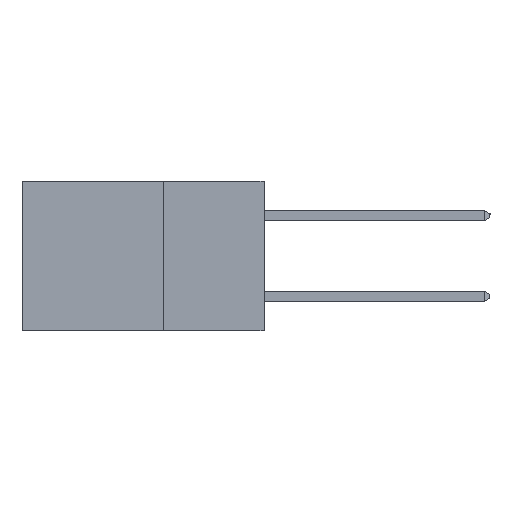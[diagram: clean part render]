
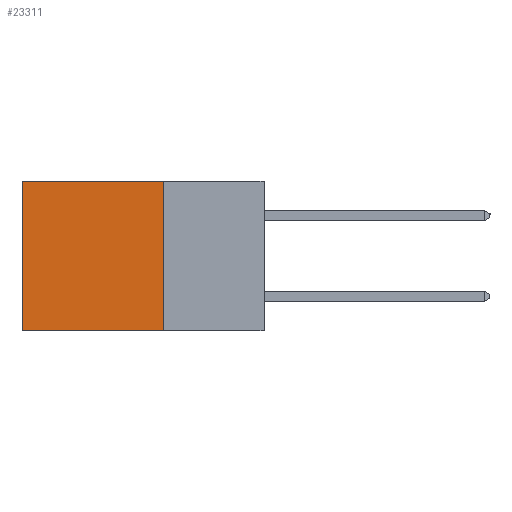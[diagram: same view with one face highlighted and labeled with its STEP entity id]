
A CAD part, left-side view. The second image highlights one B-rep face of the part: STEP entity #23311.
In plain terms, the highlighted planar face has unit normal (-1, 0, 0).
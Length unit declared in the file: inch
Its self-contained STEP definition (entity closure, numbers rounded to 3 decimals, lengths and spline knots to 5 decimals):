
#424 = CARTESIAN_POINT ( 'NONE',  ( 0.2615, 0.25, -0.37 ) ) ;
#1239 = LINE ( 'NONE', #14139, #22693 ) ;
#2942 = AXIS2_PLACEMENT_3D ( 'NONE', #22313, #9409, #12639 ) ;
#3523 = VERTEX_POINT ( 'NONE', #3964 ) ;
#3964 = CARTESIAN_POINT ( 'NONE',  ( 0.2615, 0.6, -0.37 ) ) ;
#5499 = ORIENTED_EDGE ( 'NONE', *, *, #8845, .T. ) ;
#5873 = EDGE_CURVE ( 'NONE', #17160, #3523, #1239, .T. ) ;
#6021 = LINE ( 'NONE', #424, #23474 ) ;
#7053 = DIRECTION ( 'NONE',  ( 0., 1., 0. ) ) ;
#8845 = EDGE_CURVE ( 'NONE', #20642, #14794, #18087, .T. ) ;
#8939 = PLANE ( 'NONE',  #2942 ) ;
#9409 = DIRECTION ( 'NONE',  ( 1., 0., 0. ) ) ;
#9886 = DIRECTION ( 'NONE',  ( 0., 0., -1. ) ) ;
#9913 = CARTESIAN_POINT ( 'NONE',  ( 0.2615, 0.25, -0.37 ) ) ;
#11839 = DIRECTION ( 'NONE',  ( 0., 0., -1. ) ) ;
#12007 = LINE ( 'NONE', #15729, #19194 ) ;
#12263 = EDGE_CURVE ( 'NONE', #20642, #17160, #6021, .T. ) ;
#12330 = ORIENTED_EDGE ( 'NONE', *, *, #13240, .T. ) ;
#12508 = CARTESIAN_POINT ( 'NONE',  ( 0.2615, 0.25, 0. ) ) ;
#12639 = DIRECTION ( 'NONE',  ( 0., 0., -1. ) ) ;
#13212 = VECTOR ( 'NONE', #7053, 39.37008 ) ;
#13240 = EDGE_CURVE ( 'NONE', #14794, #3523, #12007, .T. ) ;
#13629 = ORIENTED_EDGE ( 'NONE', *, *, #12263, .F. ) ;
#14024 = DIRECTION ( 'NONE',  ( 0., 1., 0. ) ) ;
#14139 = CARTESIAN_POINT ( 'NONE',  ( 0.2615, 0.25, -0.37 ) ) ;
#14794 = VERTEX_POINT ( 'NONE', #19844 ) ;
#15729 = CARTESIAN_POINT ( 'NONE',  ( 0.2615, 0.6, -0.37 ) ) ;
#17160 = VERTEX_POINT ( 'NONE', #9913 ) ;
#17414 = EDGE_LOOP ( 'NONE', ( #12330, #23998, #13629, #5499 ) ) ;
#18087 = LINE ( 'NONE', #12508, #13212 ) ;
#19194 = VECTOR ( 'NONE', #9886, 39.37008 ) ;
#19844 = CARTESIAN_POINT ( 'NONE',  ( 0.2615, 0.6, 0. ) ) ;
#20642 = VERTEX_POINT ( 'NONE', #24476 ) ;
#20694 = FACE_OUTER_BOUND ( 'NONE', #17414, .T. ) ;
#22313 = CARTESIAN_POINT ( 'NONE',  ( 0.2615, 0.25, -0.37 ) ) ;
#22693 = VECTOR ( 'NONE', #14024, 39.37008 ) ;
#23311 = ADVANCED_FACE ( 'NONE', ( #20694 ), #8939, .F. ) ;
#23474 = VECTOR ( 'NONE', #11839, 39.37008 ) ;
#23998 = ORIENTED_EDGE ( 'NONE', *, *, #5873, .F. ) ;
#24476 = CARTESIAN_POINT ( 'NONE',  ( 0.2615, 0.25, 0. ) ) ;
